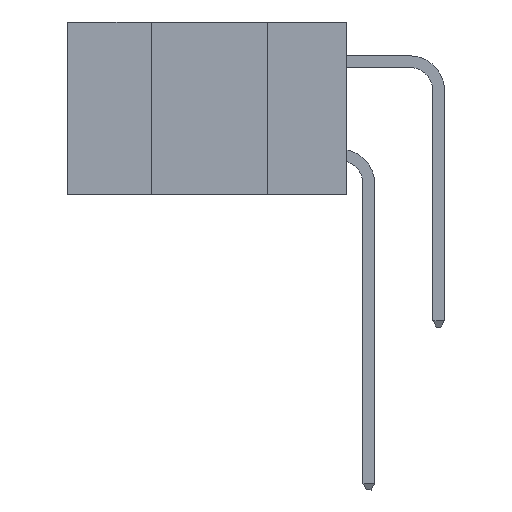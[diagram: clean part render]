
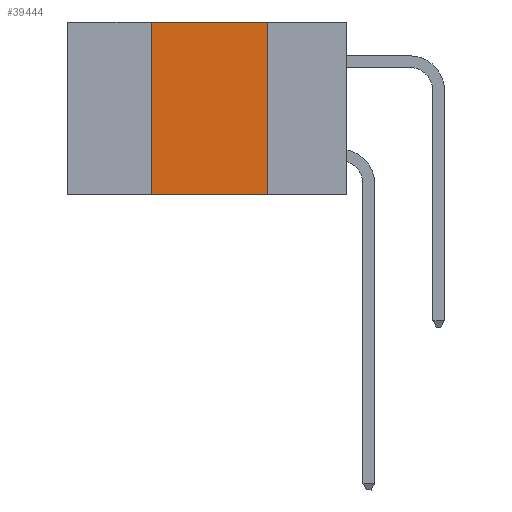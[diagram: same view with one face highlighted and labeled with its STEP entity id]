
A CAD part, left-side view. The second image highlights one B-rep face of the part: STEP entity #39444.
In plain terms, the highlighted planar face has unit normal (-1, 0, 0).
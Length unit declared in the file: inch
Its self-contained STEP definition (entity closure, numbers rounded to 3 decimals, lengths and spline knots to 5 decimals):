
#2234 = CARTESIAN_POINT ( 'NONE',  ( 0., 0.6, 0. ) ) ;
#2693 = DIRECTION ( 'NONE',  ( 0., -1., 0. ) ) ;
#3187 = CARTESIAN_POINT ( 'NONE',  ( 0., 0.42, 0. ) ) ;
#3822 = VERTEX_POINT ( 'NONE', #41261 ) ;
#4490 = CARTESIAN_POINT ( 'NONE',  ( 0., 0.6, 0. ) ) ;
#6946 = ORIENTED_EDGE ( 'NONE', *, *, #42666, .T. ) ;
#7043 = ORIENTED_EDGE ( 'NONE', *, *, #32458, .F. ) ;
#8556 = DIRECTION ( 'NONE',  ( 0., 0., -1. ) ) ;
#11642 = VERTEX_POINT ( 'NONE', #41700 ) ;
#17315 = VECTOR ( 'NONE', #28069, 39.37008 ) ;
#17638 = VERTEX_POINT ( 'NONE', #3187 ) ;
#17781 = CARTESIAN_POINT ( 'NONE',  ( 0., 0.17, 0. ) ) ;
#18655 = EDGE_CURVE ( 'NONE', #36989, #11642, #36409, .T. ) ;
#18692 = DIRECTION ( 'NONE',  ( 1., 0., 0. ) ) ;
#19843 = VECTOR ( 'NONE', #8556, 39.37008 ) ;
#20123 = AXIS2_PLACEMENT_3D ( 'NONE', #4490, #18692, #25173 ) ;
#21515 = EDGE_LOOP ( 'NONE', ( #28239, #27651, #7043, #6946 ) ) ;
#25173 = DIRECTION ( 'NONE',  ( 0., 0., -1. ) ) ;
#26009 = VECTOR ( 'NONE', #2693, 39.37008 ) ;
#27651 = ORIENTED_EDGE ( 'NONE', *, *, #34888, .F. ) ;
#28069 = DIRECTION ( 'NONE',  ( 0., 0., 1. ) ) ;
#28239 = ORIENTED_EDGE ( 'NONE', *, *, #18655, .F. ) ;
#28507 = DIRECTION ( 'NONE',  ( 0., -1., 0. ) ) ;
#29689 = CARTESIAN_POINT ( 'NONE',  ( 0., 0.17, 0. ) ) ;
#32458 = EDGE_CURVE ( 'NONE', #3822, #17638, #41638, .T. ) ;
#34888 = EDGE_CURVE ( 'NONE', #17638, #36989, #35891, .T. ) ;
#35184 = CARTESIAN_POINT ( 'NONE',  ( 0., 0.42, 0. ) ) ;
#35450 = CARTESIAN_POINT ( 'NONE',  ( 0., 0.6, -0.37 ) ) ;
#35891 = LINE ( 'NONE', #2234, #26009 ) ;
#36138 = PLANE ( 'NONE',  #20123 ) ;
#36409 = LINE ( 'NONE', #29689, #19843 ) ;
#36989 = VERTEX_POINT ( 'NONE', #17781 ) ;
#39396 = VECTOR ( 'NONE', #28507, 39.37008 ) ;
#39444 = ADVANCED_FACE ( 'NONE', ( #41900 ), #36138, .F. ) ;
#40518 = LINE ( 'NONE', #35450, #39396 ) ;
#41261 = CARTESIAN_POINT ( 'NONE',  ( 0., 0.42, -0.37 ) ) ;
#41638 = LINE ( 'NONE', #35184, #17315 ) ;
#41700 = CARTESIAN_POINT ( 'NONE',  ( 0., 0.17, -0.37 ) ) ;
#41900 = FACE_OUTER_BOUND ( 'NONE', #21515, .T. ) ;
#42666 = EDGE_CURVE ( 'NONE', #3822, #11642, #40518, .T. ) ;
